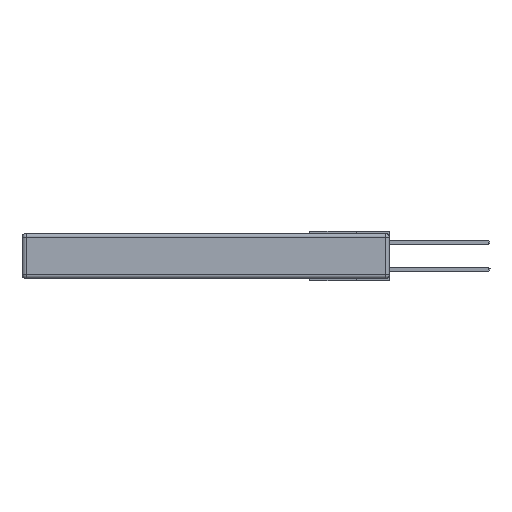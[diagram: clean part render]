
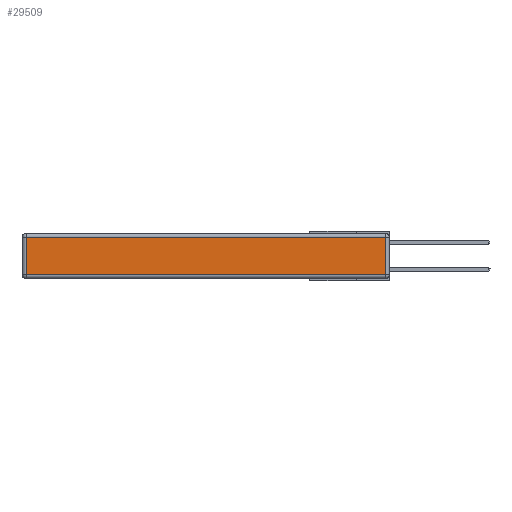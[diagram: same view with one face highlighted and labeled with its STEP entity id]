
A CAD part, left-side view. The second image highlights one B-rep face of the part: STEP entity #29509.
In plain terms, the highlighted planar face has unit normal (-1, 0, 0).
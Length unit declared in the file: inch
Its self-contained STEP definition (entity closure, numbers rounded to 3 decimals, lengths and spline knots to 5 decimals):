
#1075 = LINE ( 'NONE', #25374, #16284 ) ;
#2121 = PLANE ( 'NONE',  #5075 ) ;
#2393 = DIRECTION ( 'NONE',  ( 0., 0., -1. ) ) ;
#4838 = CARTESIAN_POINT ( 'NONE',  ( 0., 2.72, -0.313 ) ) ;
#5041 = DIRECTION ( 'NONE',  ( 0., 1., 0. ) ) ;
#5075 = AXIS2_PLACEMENT_3D ( 'NONE', #7384, #12432, #30405 ) ;
#6732 = LINE ( 'NONE', #26104, #17126 ) ;
#7384 = CARTESIAN_POINT ( 'NONE',  ( 0., 0., -0.343 ) ) ;
#9464 = EDGE_CURVE ( 'NONE', #14394, #15184, #28531, .T. ) ;
#11013 = LINE ( 'NONE', #12278, #33104 ) ;
#12055 = EDGE_CURVE ( 'NONE', #21526, #14394, #11013, .T. ) ;
#12278 = CARTESIAN_POINT ( 'NONE',  ( 0., 2.72, -0.343 ) ) ;
#12432 = DIRECTION ( 'NONE',  ( -1., 0., 0. ) ) ;
#13773 = CARTESIAN_POINT ( 'NONE',  ( 0., 0.03, -0.03 ) ) ;
#14394 = VERTEX_POINT ( 'NONE', #4838 ) ;
#14609 = CARTESIAN_POINT ( 'NONE',  ( 0., 0.03, -0.313 ) ) ;
#15184 = VERTEX_POINT ( 'NONE', #14609 ) ;
#16284 = VECTOR ( 'NONE', #5041, 39.37008 ) ;
#16335 = ORIENTED_EDGE ( 'NONE', *, *, #9464, .T. ) ;
#17126 = VECTOR ( 'NONE', #31258, 39.37008 ) ;
#17649 = EDGE_LOOP ( 'NONE', ( #16335, #22538, #23810, #22725 ) ) ;
#18420 = CARTESIAN_POINT ( 'NONE',  ( 0., 2.72, -0.03 ) ) ;
#18841 = FACE_OUTER_BOUND ( 'NONE', #17649, .T. ) ;
#19314 = EDGE_CURVE ( 'NONE', #15184, #29221, #6732, .T. ) ;
#19913 = EDGE_CURVE ( 'NONE', #29221, #21526, #1075, .T. ) ;
#21526 = VERTEX_POINT ( 'NONE', #18420 ) ;
#22538 = ORIENTED_EDGE ( 'NONE', *, *, #19314, .T. ) ;
#22725 = ORIENTED_EDGE ( 'NONE', *, *, #12055, .T. ) ;
#23700 = VECTOR ( 'NONE', #26139, 39.37008 ) ;
#23810 = ORIENTED_EDGE ( 'NONE', *, *, #19913, .T. ) ;
#25374 = CARTESIAN_POINT ( 'NONE',  ( 0., 2.75, -0.03 ) ) ;
#26104 = CARTESIAN_POINT ( 'NONE',  ( 0., 0.03, -0.343 ) ) ;
#26139 = DIRECTION ( 'NONE',  ( 0., -1., 0. ) ) ;
#28531 = LINE ( 'NONE', #28841, #23700 ) ;
#28841 = CARTESIAN_POINT ( 'NONE',  ( 0., 0., -0.313 ) ) ;
#29221 = VERTEX_POINT ( 'NONE', #13773 ) ;
#29509 = ADVANCED_FACE ( 'NONE', ( #18841 ), #2121, .T. ) ;
#30405 = DIRECTION ( 'NONE',  ( 0., 0., 1. ) ) ;
#31258 = DIRECTION ( 'NONE',  ( 0., 0., 1. ) ) ;
#33104 = VECTOR ( 'NONE', #2393, 39.37008 ) ;
